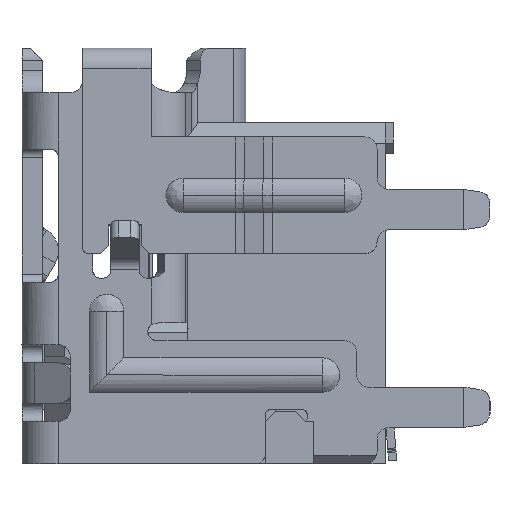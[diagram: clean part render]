
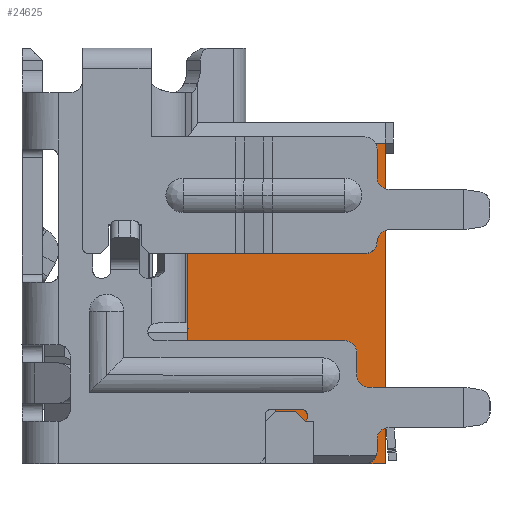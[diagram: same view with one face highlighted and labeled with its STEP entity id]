
A CAD part, left-side view. The second image highlights one B-rep face of the part: STEP entity #24625.
In plain terms, the highlighted planar face has unit normal (-1, 0, 0).
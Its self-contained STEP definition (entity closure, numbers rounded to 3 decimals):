
#2882 = ORIENTED_EDGE ( 'NONE', *, *, #14356, .F. ) ;
#3507 = VERTEX_POINT ( 'NONE', #40176 ) ;
#6218 = VECTOR ( 'NONE', #18323, 1000. ) ;
#7718 = ORIENTED_EDGE ( 'NONE', *, *, #60527, .T. ) ;
#7897 = DIRECTION ( 'NONE',  ( 0., -1., 0. ) ) ;
#9834 = LINE ( 'NONE', #10339, #6218 ) ;
#10339 = CARTESIAN_POINT ( 'NONE',  ( -6.95, -6.025, -6.5 ) ) ;
#10566 = CARTESIAN_POINT ( 'NONE',  ( -6.95, -6.025, -7.8 ) ) ;
#10795 = ORIENTED_EDGE ( 'NONE', *, *, #73520, .F. ) ;
#11634 = EDGE_LOOP ( 'NONE', ( #17943, #2882, #12145, #54902, #7718, #48639, #83853, #50947, #17646, #10795 ) ) ;
#12145 = ORIENTED_EDGE ( 'NONE', *, *, #13613, .F. ) ;
#12889 = DIRECTION ( 'NONE',  ( 0., 0., 1. ) ) ;
#12974 = CARTESIAN_POINT ( 'NONE',  ( -6.95, -8.475, -7.8 ) ) ;
#13613 = EDGE_CURVE ( 'NONE', #71988, #86796, #43101, .T. ) ;
#14231 = DIRECTION ( 'NONE',  ( 0., 0., 1. ) ) ;
#14356 = EDGE_CURVE ( 'NONE', #86796, #40108, #97882, .T. ) ;
#14470 = VECTOR ( 'NONE', #40790, 1000. ) ;
#17235 = VERTEX_POINT ( 'NONE', #87948 ) ;
#17646 = ORIENTED_EDGE ( 'NONE', *, *, #64758, .F. ) ;
#17943 = ORIENTED_EDGE ( 'NONE', *, *, #19493, .F. ) ;
#18323 = DIRECTION ( 'NONE',  ( 0., 1., 0. ) ) ;
#19121 = CARTESIAN_POINT ( 'NONE',  ( -6.95, -5.75, -3.825 ) ) ;
#19493 = EDGE_CURVE ( 'NONE', #40108, #17235, #9834, .T. ) ;
#20564 = LINE ( 'NONE', #19121, #75613 ) ;
#23795 = DIRECTION ( 'NONE',  ( 1., 0., 0. ) ) ;
#24625 = ADVANCED_FACE ( 'NONE', ( #76964 ), #83450, .F. ) ;
#24854 = CARTESIAN_POINT ( 'NONE',  ( -6.95, -6.025, 0.15 ) ) ;
#29810 = CARTESIAN_POINT ( 'NONE',  ( -6.95, -6.5, -6.75 ) ) ;
#30551 = AXIS2_PLACEMENT_3D ( 'NONE', #58725, #23795, #7897 ) ;
#32047 = DIRECTION ( 'NONE',  ( 0., 0., -1. ) ) ;
#32434 = DIRECTION ( 'NONE',  ( 0., 1., 0. ) ) ;
#32470 = VECTOR ( 'NONE', #14231, 1000. ) ;
#33321 = LINE ( 'NONE', #39300, #14470 ) ;
#34598 = VERTEX_POINT ( 'NONE', #12974 ) ;
#34789 = CARTESIAN_POINT ( 'NONE',  ( -6.95, -8.475, -3.575 ) ) ;
#34891 = EDGE_CURVE ( 'NONE', #63527, #3507, #92933, .T. ) ;
#37955 = VERTEX_POINT ( 'NONE', #72404 ) ;
#39300 = CARTESIAN_POINT ( 'NONE',  ( -6.95, -6.025, -6.2 ) ) ;
#40108 = VERTEX_POINT ( 'NONE', #59215 ) ;
#40176 = CARTESIAN_POINT ( 'NONE',  ( -6.95, -8.475, 0.15 ) ) ;
#40790 = DIRECTION ( 'NONE',  ( 0., 1., 0. ) ) ;
#41018 = LINE ( 'NONE', #92676, #55538 ) ;
#42080 = VECTOR ( 'NONE', #97383, 1000. ) ;
#43101 = LINE ( 'NONE', #81349, #32470 ) ;
#45417 = VECTOR ( 'NONE', #32434, 1000. ) ;
#48639 = ORIENTED_EDGE ( 'NONE', *, *, #34891, .F. ) ;
#48778 = DIRECTION ( 'NONE',  ( 0., 0., 1. ) ) ;
#49194 = LINE ( 'NONE', #34789, #63198 ) ;
#49372 = DIRECTION ( 'NONE',  ( 0., 0., 1. ) ) ;
#50947 = ORIENTED_EDGE ( 'NONE', *, *, #51935, .T. ) ;
#51935 = EDGE_CURVE ( 'NONE', #37955, #61671, #41018, .T. ) ;
#54902 = ORIENTED_EDGE ( 'NONE', *, *, #85538, .F. ) ;
#55482 = CARTESIAN_POINT ( 'NONE',  ( -6.95, -6.5, -7.8 ) ) ;
#55538 = VECTOR ( 'NONE', #32047, 1000. ) ;
#58725 = CARTESIAN_POINT ( 'NONE',  ( -6.95, -3.477, 0.309 ) ) ;
#59215 = CARTESIAN_POINT ( 'NONE',  ( -6.95, -6.25, -6.5 ) ) ;
#60527 = EDGE_CURVE ( 'NONE', #34598, #3507, #49194, .T. ) ;
#61671 = VERTEX_POINT ( 'NONE', #70966 ) ;
#63198 = VECTOR ( 'NONE', #12889, 1000. ) ;
#63527 = VERTEX_POINT ( 'NONE', #89641 ) ;
#64758 = EDGE_CURVE ( 'NONE', #78119, #61671, #33321, .T. ) ;
#65171 = CARTESIAN_POINT ( 'NONE',  ( -6.95, -3.575, -3.825 ) ) ;
#69736 = LINE ( 'NONE', #10566, #45417 ) ;
#70966 = CARTESIAN_POINT ( 'NONE',  ( -6.95, -3.575, -6.2 ) ) ;
#71988 = VERTEX_POINT ( 'NONE', #55482 ) ;
#72404 = CARTESIAN_POINT ( 'NONE',  ( -6.95, -3.575, -4.5 ) ) ;
#73520 = EDGE_CURVE ( 'NONE', #17235, #78119, #20564, .T. ) ;
#75613 = VECTOR ( 'NONE', #49372, 1000. ) ;
#76964 = FACE_OUTER_BOUND ( 'NONE', #11634, .T. ) ;
#77195 = EDGE_CURVE ( 'NONE', #37955, #63527, #87061, .T. ) ;
#78119 = VERTEX_POINT ( 'NONE', #91173 ) ;
#81349 = CARTESIAN_POINT ( 'NONE',  ( -6.95, -6.5, -3.825 ) ) ;
#83450 = PLANE ( 'NONE',  #30551 ) ;
#83853 = ORIENTED_EDGE ( 'NONE', *, *, #77195, .F. ) ;
#85506 = DIRECTION ( 'NONE',  ( 0., -1., 0. ) ) ;
#85538 = EDGE_CURVE ( 'NONE', #34598, #71988, #69736, .T. ) ;
#86796 = VERTEX_POINT ( 'NONE', #96034 ) ;
#87061 = LINE ( 'NONE', #65171, #87095 ) ;
#87095 = VECTOR ( 'NONE', #48778, 1000. ) ;
#87948 = CARTESIAN_POINT ( 'NONE',  ( -6.95, -5.75, -6.5 ) ) ;
#89641 = CARTESIAN_POINT ( 'NONE',  ( -6.95, -3.575, 0.15 ) ) ;
#91173 = CARTESIAN_POINT ( 'NONE',  ( -6.95, -5.75, -6.2 ) ) ;
#92676 = CARTESIAN_POINT ( 'NONE',  ( -6.95, -3.575, -5.4 ) ) ;
#92933 = LINE ( 'NONE', #24854, #97611 ) ;
#96034 = CARTESIAN_POINT ( 'NONE',  ( -6.95, -6.5, -6.75 ) ) ;
#97383 = DIRECTION ( 'NONE',  ( 0., 0.707, 0.707 ) ) ;
#97611 = VECTOR ( 'NONE', #85506, 1000. ) ;
#97882 = LINE ( 'NONE', #29810, #42080 ) ;
